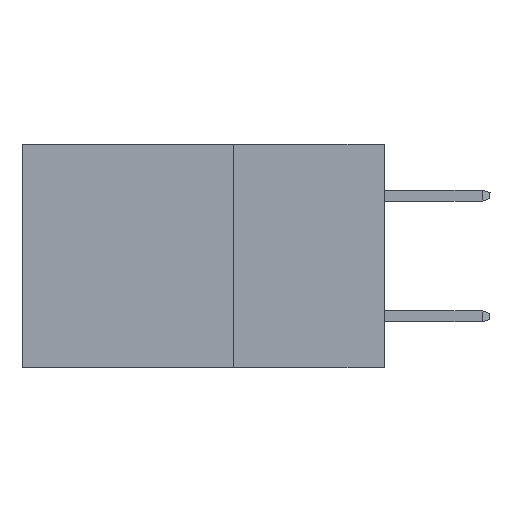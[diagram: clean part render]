
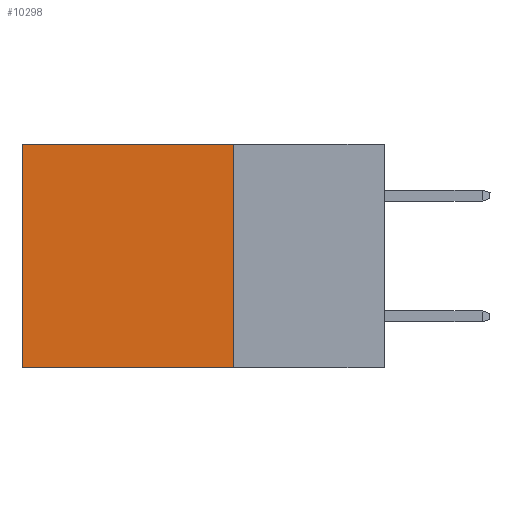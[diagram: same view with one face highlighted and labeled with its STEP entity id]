
A CAD part, left-side view. The second image highlights one B-rep face of the part: STEP entity #10298.
In plain terms, the highlighted planar face has unit normal (-1, 0, 0).
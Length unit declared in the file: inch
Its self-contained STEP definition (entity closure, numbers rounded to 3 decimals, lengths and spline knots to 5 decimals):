
#219 = CARTESIAN_POINT ( 'NONE',  ( 0.298, 0.6, 0. ) ) ;
#2581 = CARTESIAN_POINT ( 'NONE',  ( 0.298, 0.6, -0.37 ) ) ;
#2863 = DIRECTION ( 'NONE',  ( 0., 1., 0. ) ) ;
#3308 = CARTESIAN_POINT ( 'NONE',  ( 0.298, 0.25, 0. ) ) ;
#4276 = VECTOR ( 'NONE', #6187, 39.37008 ) ;
#6151 = CARTESIAN_POINT ( 'NONE',  ( 0.298, 0.25, 0. ) ) ;
#6187 = DIRECTION ( 'NONE',  ( 0., 1., 0. ) ) ;
#7216 = ORIENTED_EDGE ( 'NONE', *, *, #9739, .T. ) ;
#7328 = DIRECTION ( 'NONE',  ( 0., 0., -1. ) ) ;
#7584 = DIRECTION ( 'NONE',  ( 1., 0., 0. ) ) ;
#8963 = LINE ( 'NONE', #23152, #4276 ) ;
#9739 = EDGE_CURVE ( 'NONE', #13907, #17933, #21834, .T. ) ;
#10205 = EDGE_LOOP ( 'NONE', ( #22638, #21710, #15646, #7216 ) ) ;
#10298 = ADVANCED_FACE ( 'NONE', ( #18761 ), #24474, .F. ) ;
#10402 = AXIS2_PLACEMENT_3D ( 'NONE', #3308, #7584, #7328 ) ;
#11561 = VECTOR ( 'NONE', #2863, 39.37008 ) ;
#12641 = VECTOR ( 'NONE', #22842, 39.37008 ) ;
#13445 = CARTESIAN_POINT ( 'NONE',  ( 0.298, 0.6, 0. ) ) ;
#13623 = EDGE_CURVE ( 'NONE', #17933, #23737, #14247, .T. ) ;
#13907 = VERTEX_POINT ( 'NONE', #24302 ) ;
#14247 = LINE ( 'NONE', #219, #24833 ) ;
#15646 = ORIENTED_EDGE ( 'NONE', *, *, #24473, .F. ) ;
#17933 = VERTEX_POINT ( 'NONE', #13445 ) ;
#17984 = CARTESIAN_POINT ( 'NONE',  ( 0.298, 0.25, -0.37 ) ) ;
#18761 = FACE_OUTER_BOUND ( 'NONE', #10205, .T. ) ;
#21380 = DIRECTION ( 'NONE',  ( 0., 0., -1. ) ) ;
#21710 = ORIENTED_EDGE ( 'NONE', *, *, #22978, .F. ) ;
#21834 = LINE ( 'NONE', #25888, #11561 ) ;
#22638 = ORIENTED_EDGE ( 'NONE', *, *, #13623, .T. ) ;
#22842 = DIRECTION ( 'NONE',  ( 0., 0., -1. ) ) ;
#22978 = EDGE_CURVE ( 'NONE', #23598, #23737, #8963, .T. ) ;
#23152 = CARTESIAN_POINT ( 'NONE',  ( 0.298, 0.25, -0.37 ) ) ;
#23236 = LINE ( 'NONE', #6151, #12641 ) ;
#23598 = VERTEX_POINT ( 'NONE', #17984 ) ;
#23737 = VERTEX_POINT ( 'NONE', #2581 ) ;
#24302 = CARTESIAN_POINT ( 'NONE',  ( 0.298, 0.25, 0. ) ) ;
#24473 = EDGE_CURVE ( 'NONE', #13907, #23598, #23236, .T. ) ;
#24474 = PLANE ( 'NONE',  #10402 ) ;
#24833 = VECTOR ( 'NONE', #21380, 39.37008 ) ;
#25888 = CARTESIAN_POINT ( 'NONE',  ( 0.298, 0.25, 0. ) ) ;
